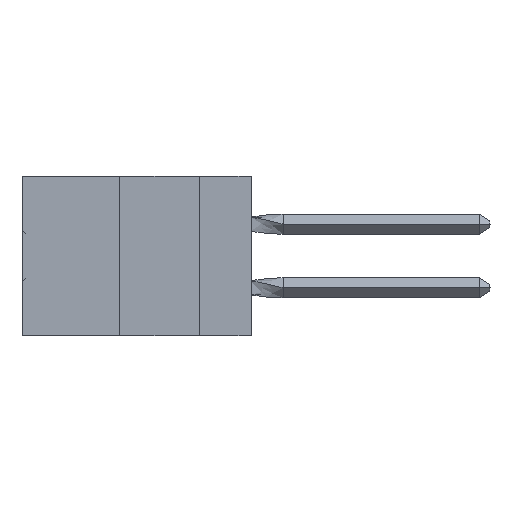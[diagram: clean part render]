
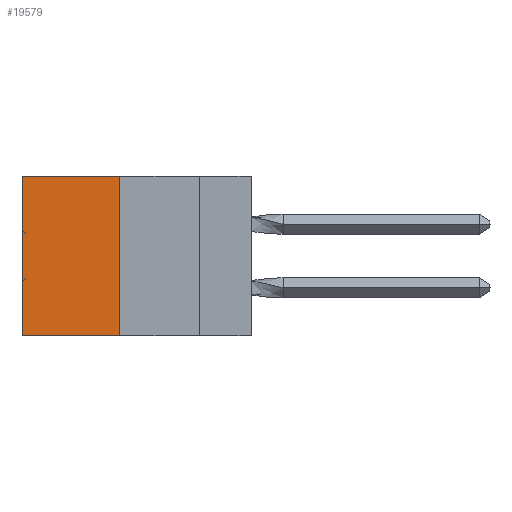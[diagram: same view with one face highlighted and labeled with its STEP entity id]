
A CAD part, left-side view. The second image highlights one B-rep face of the part: STEP entity #19579.
In plain terms, the highlighted planar face has unit normal (-1, 0, 0).
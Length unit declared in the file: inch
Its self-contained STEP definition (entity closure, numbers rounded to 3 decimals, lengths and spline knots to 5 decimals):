
#467 = CARTESIAN_POINT ( 'NONE',  ( 0.305, 0.72, 0. ) ) ;
#2365 = PLANE ( 'NONE',  #45268 ) ;
#3038 = DIRECTION ( 'NONE',  ( 0., 1., 0. ) ) ;
#3319 = ORIENTED_EDGE ( 'NONE', *, *, #50877, .F. ) ;
#5051 = EDGE_LOOP ( 'NONE', ( #15682, #3319, #8110, #53297 ) ) ;
#7114 = CARTESIAN_POINT ( 'NONE',  ( 0.305, 0.72, -0.5 ) ) ;
#7850 = CARTESIAN_POINT ( 'NONE',  ( 0.305, 0.413, 0. ) ) ;
#8110 = ORIENTED_EDGE ( 'NONE', *, *, #30550, .F. ) ;
#9029 = CARTESIAN_POINT ( 'NONE',  ( 0.305, 0.413, -0.5 ) ) ;
#9856 = LINE ( 'NONE', #23770, #51178 ) ;
#10429 = CARTESIAN_POINT ( 'NONE',  ( 0.305, 0.413, -0.5 ) ) ;
#12121 = DIRECTION ( 'NONE',  ( 0., 0., -1. ) ) ;
#13410 = DIRECTION ( 'NONE',  ( 0., 0., -1. ) ) ;
#14726 = CARTESIAN_POINT ( 'NONE',  ( 0.305, 0.413, -0.5 ) ) ;
#15682 = ORIENTED_EDGE ( 'NONE', *, *, #35914, .T. ) ;
#16459 = VERTEX_POINT ( 'NONE', #7114 ) ;
#16655 = VECTOR ( 'NONE', #13410, 39.37008 ) ;
#17439 = VERTEX_POINT ( 'NONE', #41395 ) ;
#19579 = ADVANCED_FACE ( 'NONE', ( #23203 ), #2365, .F. ) ;
#20090 = LINE ( 'NONE', #9029, #16655 ) ;
#21562 = VECTOR ( 'NONE', #28494, 39.37008 ) ;
#23203 = FACE_OUTER_BOUND ( 'NONE', #5051, .T. ) ;
#23590 = DIRECTION ( 'NONE',  ( 0., 0., -1. ) ) ;
#23770 = CARTESIAN_POINT ( 'NONE',  ( 0.305, 0.72, -0.5 ) ) ;
#27729 = VERTEX_POINT ( 'NONE', #467 ) ;
#28494 = DIRECTION ( 'NONE',  ( 0., 1., 0. ) ) ;
#28538 = DIRECTION ( 'NONE',  ( 1., 0., 0. ) ) ;
#30550 = EDGE_CURVE ( 'NONE', #17439, #36942, #20090, .T. ) ;
#35914 = EDGE_CURVE ( 'NONE', #27729, #16459, #9856, .T. ) ;
#36942 = VERTEX_POINT ( 'NONE', #14726 ) ;
#41395 = CARTESIAN_POINT ( 'NONE',  ( 0.305, 0.413, 0. ) ) ;
#42626 = EDGE_CURVE ( 'NONE', #17439, #27729, #56272, .T. ) ;
#44607 = VECTOR ( 'NONE', #3038, 39.37008 ) ;
#45268 = AXIS2_PLACEMENT_3D ( 'NONE', #54890, #28538, #12121 ) ;
#50559 = LINE ( 'NONE', #10429, #21562 ) ;
#50877 = EDGE_CURVE ( 'NONE', #36942, #16459, #50559, .T. ) ;
#51178 = VECTOR ( 'NONE', #23590, 39.37008 ) ;
#53297 = ORIENTED_EDGE ( 'NONE', *, *, #42626, .T. ) ;
#54890 = CARTESIAN_POINT ( 'NONE',  ( 0.305, 0.413, -0.5 ) ) ;
#56272 = LINE ( 'NONE', #7850, #44607 ) ;
